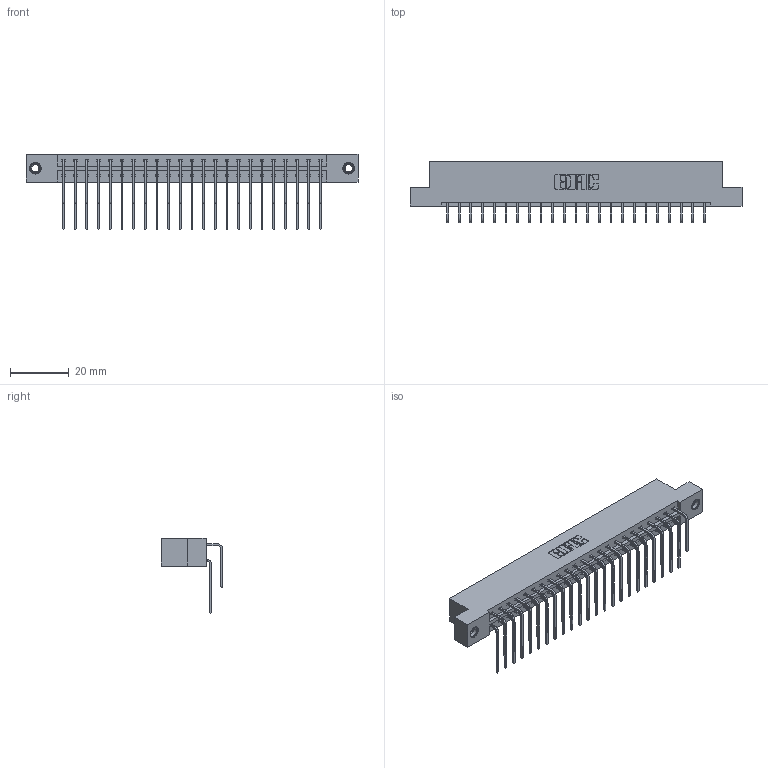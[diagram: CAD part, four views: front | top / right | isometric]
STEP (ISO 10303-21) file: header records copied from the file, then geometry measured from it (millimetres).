
FILE_DESCRIPTION (( 'STEP AP203' ), '1' );
FILE_NAME ('833-046-559-207.STEP', '2020-06-04T15:05:32', ( '' ), ( '' ), 'SwSTEP 2.0', 'SolidWorks 2020', '' );
FILE_SCHEMA (( 'CONFIG_CONTROL_DESIGN' ));
Length unit declared in the file: inch
Products named in the file (5): 345-250-001_345-250-005-103; 833 Part_Flush - .156 Dia - TI; 345-292-001_558 559 Tail - 1; 833-046-559-207; 345-292-001_559 Tail - 2
Assembly tree (49 placements, depth 2):
  833-046-559-207
    833 Part_Flush - .156 Dia - TI
    345-292-001_558 559 Tail - 1  x23
    345-292-001_559 Tail - 2  x23
    345-250-001_345-250-005-103  x2
Bounding box: 112.67 x 20.9 x 25.53 mm (x, y, z)
Volume: 11577.6 mm3; surface area: 14839.3 mm2
Topology: 49 solids, 49 shells, 2658 faces, 7853 edges, 5166 vertices
Faces by surface type: plane 1850, cylinder 792, cone 12, torus 4
Entity records: 20224 total; most frequent: CARTESIAN_POINT 3408, ORIENTED_EDGE 3286, DIRECTION 2957, EDGE_CURVE 1643, VECTOR 1455, LINE 1455, VERTEX_POINT 1088, AXIS2_PLACEMENT_3D 751
